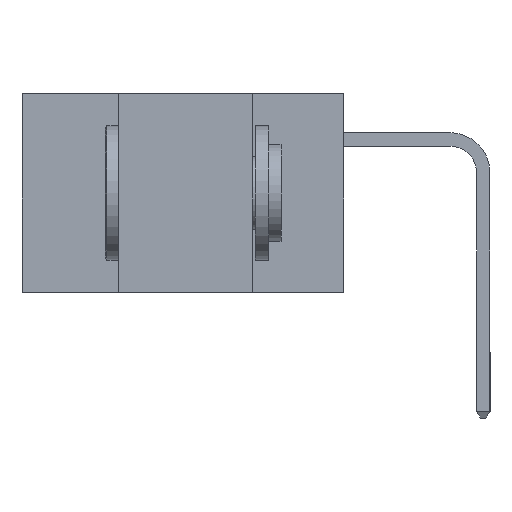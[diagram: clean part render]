
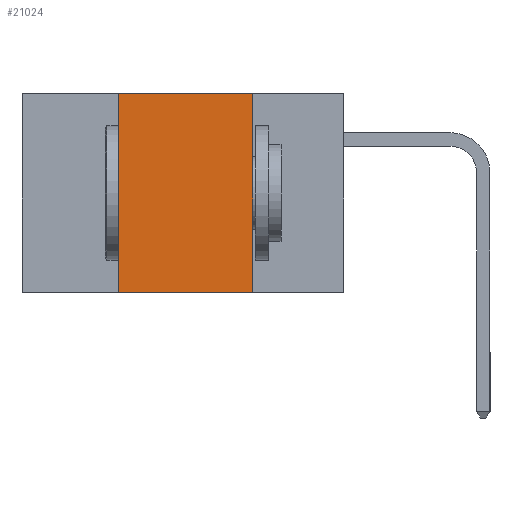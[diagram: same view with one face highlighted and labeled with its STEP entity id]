
A CAD part, left-side view. The second image highlights one B-rep face of the part: STEP entity #21024.
In plain terms, the highlighted planar face has unit normal (-1, 0, 0).
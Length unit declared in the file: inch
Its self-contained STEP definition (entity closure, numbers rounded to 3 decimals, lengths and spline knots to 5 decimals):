
#521 = DIRECTION ( 'NONE',  ( 0., 0., -1. ) ) ;
#1366 = VECTOR ( 'NONE', #3011, 39.37008 ) ;
#3011 = DIRECTION ( 'NONE',  ( 0., -1., 0. ) ) ;
#3902 = VERTEX_POINT ( 'NONE', #21811 ) ;
#3919 = EDGE_LOOP ( 'NONE', ( #30117, #22906, #14933, #20940 ) ) ;
#4599 = AXIS2_PLACEMENT_3D ( 'NONE', #21323, #26395, #11398 ) ;
#6788 = EDGE_CURVE ( 'NONE', #22507, #15687, #30076, .T. ) ;
#8884 = PLANE ( 'NONE',  #4599 ) ;
#10478 = CARTESIAN_POINT ( 'NONE',  ( 0., 0.17, 0. ) ) ;
#11398 = DIRECTION ( 'NONE',  ( 0., 0., -1. ) ) ;
#11563 = CARTESIAN_POINT ( 'NONE',  ( 0., 0.42, 0. ) ) ;
#12924 = CARTESIAN_POINT ( 'NONE',  ( 0., 0.6, -0.37 ) ) ;
#13131 = VERTEX_POINT ( 'NONE', #13410 ) ;
#13410 = CARTESIAN_POINT ( 'NONE',  ( 0., 0.42, -0.37 ) ) ;
#14542 = CARTESIAN_POINT ( 'NONE',  ( 0., 0.6, 0. ) ) ;
#14932 = VECTOR ( 'NONE', #521, 39.37008 ) ;
#14933 = ORIENTED_EDGE ( 'NONE', *, *, #20078, .F. ) ;
#15007 = LINE ( 'NONE', #22262, #27560 ) ;
#15687 = VERTEX_POINT ( 'NONE', #16212 ) ;
#16212 = CARTESIAN_POINT ( 'NONE',  ( 0., 0.17, 0. ) ) ;
#16866 = VECTOR ( 'NONE', #24536, 39.37008 ) ;
#20078 = EDGE_CURVE ( 'NONE', #13131, #22507, #15007, .T. ) ;
#20940 = ORIENTED_EDGE ( 'NONE', *, *, #30752, .T. ) ;
#21024 = ADVANCED_FACE ( 'NONE', ( #25195 ), #8884, .F. ) ;
#21323 = CARTESIAN_POINT ( 'NONE',  ( 0., 0.6, 0. ) ) ;
#21609 = LINE ( 'NONE', #10478, #14932 ) ;
#21811 = CARTESIAN_POINT ( 'NONE',  ( 0., 0.17, -0.37 ) ) ;
#22262 = CARTESIAN_POINT ( 'NONE',  ( 0., 0.42, 0. ) ) ;
#22507 = VERTEX_POINT ( 'NONE', #11563 ) ;
#22906 = ORIENTED_EDGE ( 'NONE', *, *, #6788, .F. ) ;
#24083 = EDGE_CURVE ( 'NONE', #15687, #3902, #21609, .T. ) ;
#24536 = DIRECTION ( 'NONE',  ( 0., -1., 0. ) ) ;
#24817 = DIRECTION ( 'NONE',  ( 0., 0., 1. ) ) ;
#25195 = FACE_OUTER_BOUND ( 'NONE', #3919, .T. ) ;
#26395 = DIRECTION ( 'NONE',  ( 1., 0., 0. ) ) ;
#27560 = VECTOR ( 'NONE', #24817, 39.37008 ) ;
#27865 = LINE ( 'NONE', #12924, #1366 ) ;
#30076 = LINE ( 'NONE', #14542, #16866 ) ;
#30117 = ORIENTED_EDGE ( 'NONE', *, *, #24083, .F. ) ;
#30752 = EDGE_CURVE ( 'NONE', #13131, #3902, #27865, .T. ) ;
